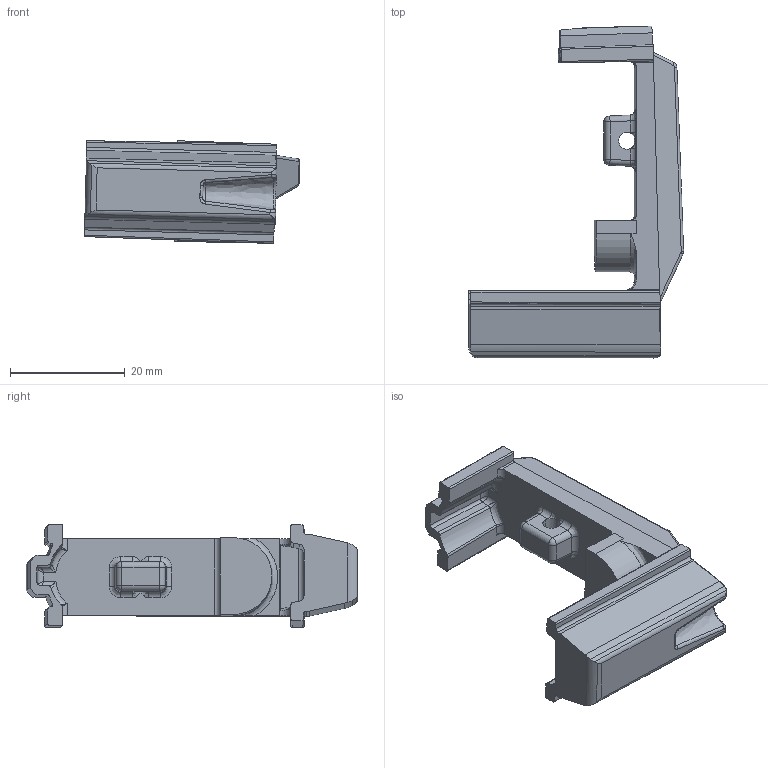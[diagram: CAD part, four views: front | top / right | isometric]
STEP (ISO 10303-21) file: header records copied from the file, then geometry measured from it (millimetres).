
FILE_DESCRIPTION (( 'STEP AP214' ), '1' );
FILE_NAME ('Follower.STEP', '2022-09-24T15:51:18', ( '' ), ( '' ), 'SwSTEP 2.0', 'SolidWorks 2021', '' );
FILE_SCHEMA (( 'AUTOMOTIVE_DESIGN' ));
Length unit declared in the file: millimetre
Products named in the file (1): Follower
Bounding box: 37.54 x 57.89 x 17.9 mm (x, y, z)
Volume: 8711.8 mm3; surface area: 4977.4 mm2
Topology: 1 solids, 1 shells, 201 faces, 547 edges, 333 vertices
Faces by surface type: bspline 73, cylinder 64, plane 57, sphere 4, torus 3
Entity records: 8182 total; most frequent: CARTESIAN_POINT 3849, ORIENTED_EDGE 1062, DIRECTION 700, EDGE_CURVE 531, VERTEX_POINT 331, AXIS2_PLACEMENT_3D 239, LINE 222, VECTOR 222
